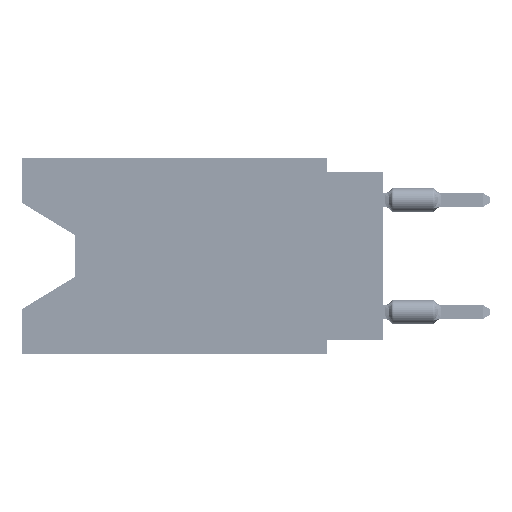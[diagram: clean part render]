
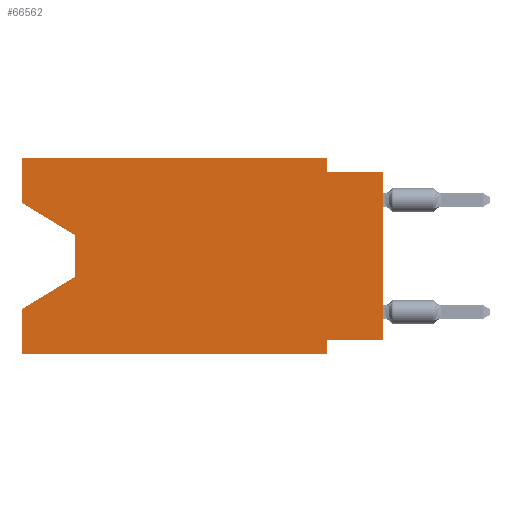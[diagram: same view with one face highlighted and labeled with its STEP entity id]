
A CAD part, left-side view. The second image highlights one B-rep face of the part: STEP entity #66562.
In plain terms, the highlighted planar face has unit normal (-1, 0, 0).
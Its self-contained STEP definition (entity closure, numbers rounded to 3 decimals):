
#141 = VECTOR ( 'NONE', #81739, 1000. ) ;
#903 = ORIENTED_EDGE ( 'NONE', *, *, #40198, .F. ) ;
#1154 = CARTESIAN_POINT ( 'NONE',  ( 0., 2.54, -8.89 ) ) ;
#3203 = ORIENTED_EDGE ( 'NONE', *, *, #39359, .F. ) ;
#3940 = LINE ( 'NONE', #42768, #35890 ) ;
#4160 = VECTOR ( 'NONE', #45078, 1000. ) ;
#4454 = LINE ( 'NONE', #24272, #12110 ) ;
#5407 = AXIS2_PLACEMENT_3D ( 'NONE', #28521, #40772, #60608 ) ;
#5945 = CARTESIAN_POINT ( 'NONE',  ( 0., 0., -0.635 ) ) ;
#7152 = LINE ( 'NONE', #57825, #47009 ) ;
#7156 = EDGE_LOOP ( 'NONE', ( #12635, #41188, #65834, #18972, #14965, #3203, #35053, #8039, #51043, #45510, #73398, #903 ) ) ;
#7430 = PLANE ( 'NONE',  #5407 ) ;
#7629 = CARTESIAN_POINT ( 'NONE',  ( 0., 13.97, -5.385 ) ) ;
#8039 = ORIENTED_EDGE ( 'NONE', *, *, #67942, .T. ) ;
#9171 = VERTEX_POINT ( 'NONE', #45917 ) ;
#9664 = CARTESIAN_POINT ( 'NONE',  ( 0., 2.54, 0. ) ) ;
#12110 = VECTOR ( 'NONE', #62675, 1000. ) ;
#12328 = LINE ( 'NONE', #38065, #30513 ) ;
#12515 = CARTESIAN_POINT ( 'NONE',  ( 0., 16.383, 0. ) ) ;
#12635 = ORIENTED_EDGE ( 'NONE', *, *, #42258, .T. ) ;
#13766 = FACE_OUTER_BOUND ( 'NONE', #7156, .T. ) ;
#14965 = ORIENTED_EDGE ( 'NONE', *, *, #76619, .T. ) ;
#16681 = EDGE_CURVE ( 'NONE', #9171, #34113, #69906, .T. ) ;
#17092 = DIRECTION ( 'NONE',  ( 0., 0., -1. ) ) ;
#17387 = VECTOR ( 'NONE', #81372, 1000. ) ;
#17789 = CARTESIAN_POINT ( 'NONE',  ( 0., 16.383, -2.038 ) ) ;
#18689 = CARTESIAN_POINT ( 'NONE',  ( 0., 16.383, 0. ) ) ;
#18972 = ORIENTED_EDGE ( 'NONE', *, *, #22159, .F. ) ;
#20895 = VERTEX_POINT ( 'NONE', #35668 ) ;
#22159 = EDGE_CURVE ( 'NONE', #72841, #20895, #70333, .T. ) ;
#24272 = CARTESIAN_POINT ( 'NONE',  ( 0., 0., 0. ) ) ;
#27846 = VECTOR ( 'NONE', #65108, 1000. ) ;
#28521 = CARTESIAN_POINT ( 'NONE',  ( 0., 16.383, 0. ) ) ;
#29511 = CARTESIAN_POINT ( 'NONE',  ( 0., 13.97, -3.505 ) ) ;
#29755 = CARTESIAN_POINT ( 'NONE',  ( 0., 16.383, 0. ) ) ;
#29889 = CARTESIAN_POINT ( 'NONE',  ( 0., 16.383, 0. ) ) ;
#30183 = LINE ( 'NONE', #55925, #46097 ) ;
#30513 = VECTOR ( 'NONE', #52401, 1000. ) ;
#30611 = EDGE_CURVE ( 'NONE', #46464, #31199, #32093, .T. ) ;
#31199 = VERTEX_POINT ( 'NONE', #71236 ) ;
#32093 = LINE ( 'NONE', #5945, #69205 ) ;
#34113 = VERTEX_POINT ( 'NONE', #78077 ) ;
#34426 = CARTESIAN_POINT ( 'NONE',  ( 0., 13.97, -5.385 ) ) ;
#35053 = ORIENTED_EDGE ( 'NONE', *, *, #16681, .F. ) ;
#35668 = CARTESIAN_POINT ( 'NONE',  ( 0., 16.383, -6.852 ) ) ;
#35890 = VECTOR ( 'NONE', #55004, 1000. ) ;
#36153 = CARTESIAN_POINT ( 'NONE',  ( 0., 2.54, -0.635 ) ) ;
#37986 = VERTEX_POINT ( 'NONE', #9664 ) ;
#38065 = CARTESIAN_POINT ( 'NONE',  ( 0., 2.54, 0. ) ) ;
#39359 = EDGE_CURVE ( 'NONE', #34113, #51740, #65719, .T. ) ;
#40198 = EDGE_CURVE ( 'NONE', #59708, #53291, #58367, .T. ) ;
#40772 = DIRECTION ( 'NONE',  ( 1., 0., 0. ) ) ;
#41188 = ORIENTED_EDGE ( 'NONE', *, *, #55056, .T. ) ;
#41262 = EDGE_CURVE ( 'NONE', #59780, #20895, #49186, .T. ) ;
#42258 = EDGE_CURVE ( 'NONE', #59708, #47620, #7152, .T. ) ;
#42768 = CARTESIAN_POINT ( 'NONE',  ( 0., 16.383, -8.89 ) ) ;
#45078 = DIRECTION ( 'NONE',  ( 0., 0., -1. ) ) ;
#45510 = ORIENTED_EDGE ( 'NONE', *, *, #77263, .F. ) ;
#45917 = CARTESIAN_POINT ( 'NONE',  ( 0., 0., -8.255 ) ) ;
#46097 = VECTOR ( 'NONE', #17092, 1000. ) ;
#46464 = VERTEX_POINT ( 'NONE', #36153 ) ;
#47009 = VECTOR ( 'NONE', #63735, 1000. ) ;
#47620 = VERTEX_POINT ( 'NONE', #29511 ) ;
#49186 = LINE ( 'NONE', #34426, #72486 ) ;
#50614 = EDGE_CURVE ( 'NONE', #53291, #37986, #56888, .T. ) ;
#51043 = ORIENTED_EDGE ( 'NONE', *, *, #30611, .F. ) ;
#51740 = VERTEX_POINT ( 'NONE', #79000 ) ;
#52401 = DIRECTION ( 'NONE',  ( 0., 0., -1. ) ) ;
#53291 = VERTEX_POINT ( 'NONE', #29755 ) ;
#55004 = DIRECTION ( 'NONE',  ( 0., -1., 0. ) ) ;
#55056 = EDGE_CURVE ( 'NONE', #47620, #59780, #30183, .T. ) ;
#55584 = CARTESIAN_POINT ( 'NONE',  ( 0., 0., -8.255 ) ) ;
#55925 = CARTESIAN_POINT ( 'NONE',  ( 0., 13.97, -3.505 ) ) ;
#56888 = LINE ( 'NONE', #29889, #17387 ) ;
#57825 = CARTESIAN_POINT ( 'NONE',  ( 0., 16.383, -2.038 ) ) ;
#58367 = LINE ( 'NONE', #18689, #27846 ) ;
#59708 = VERTEX_POINT ( 'NONE', #17789 ) ;
#59780 = VERTEX_POINT ( 'NONE', #7629 ) ;
#60608 = DIRECTION ( 'NONE',  ( 0., 0., -1. ) ) ;
#60614 = DIRECTION ( 'NONE',  ( 0., 0.855, -0.519 ) ) ;
#62443 = CARTESIAN_POINT ( 'NONE',  ( 0., 16.383, -8.89 ) ) ;
#62675 = DIRECTION ( 'NONE',  ( 0., 0., 1. ) ) ;
#63735 = DIRECTION ( 'NONE',  ( 0., -0.855, -0.519 ) ) ;
#63994 = DIRECTION ( 'NONE',  ( 0., 0., 1. ) ) ;
#65108 = DIRECTION ( 'NONE',  ( 0., 0., 1. ) ) ;
#65719 = LINE ( 'NONE', #1154, #4160 ) ;
#65834 = ORIENTED_EDGE ( 'NONE', *, *, #41262, .T. ) ;
#66562 = ADVANCED_FACE ( 'NONE', ( #13766 ), #7430, .F. ) ;
#67942 = EDGE_CURVE ( 'NONE', #9171, #31199, #4454, .T. ) ;
#69205 = VECTOR ( 'NONE', #81911, 1000. ) ;
#69906 = LINE ( 'NONE', #55584, #141 ) ;
#70333 = LINE ( 'NONE', #12515, #74909 ) ;
#71236 = CARTESIAN_POINT ( 'NONE',  ( 0., 0., -0.635 ) ) ;
#72486 = VECTOR ( 'NONE', #60614, 1000. ) ;
#72841 = VERTEX_POINT ( 'NONE', #62443 ) ;
#73398 = ORIENTED_EDGE ( 'NONE', *, *, #50614, .F. ) ;
#74909 = VECTOR ( 'NONE', #63994, 1000. ) ;
#76619 = EDGE_CURVE ( 'NONE', #72841, #51740, #3940, .T. ) ;
#77263 = EDGE_CURVE ( 'NONE', #37986, #46464, #12328, .T. ) ;
#78077 = CARTESIAN_POINT ( 'NONE',  ( 0., 2.54, -8.255 ) ) ;
#79000 = CARTESIAN_POINT ( 'NONE',  ( 0., 2.54, -8.89 ) ) ;
#81372 = DIRECTION ( 'NONE',  ( 0., -1., 0. ) ) ;
#81739 = DIRECTION ( 'NONE',  ( 0., 1., 0. ) ) ;
#81911 = DIRECTION ( 'NONE',  ( 0., -1., 0. ) ) ;
